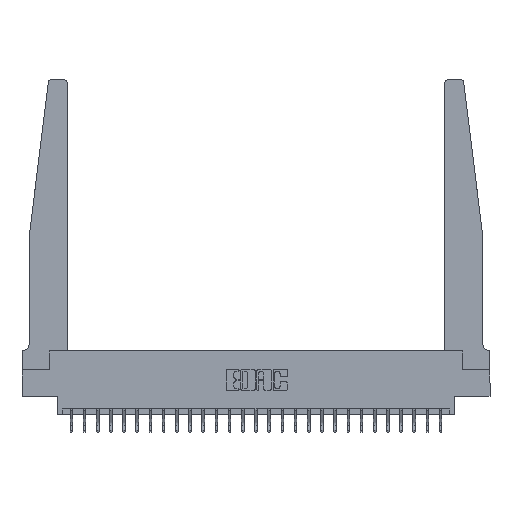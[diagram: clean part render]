
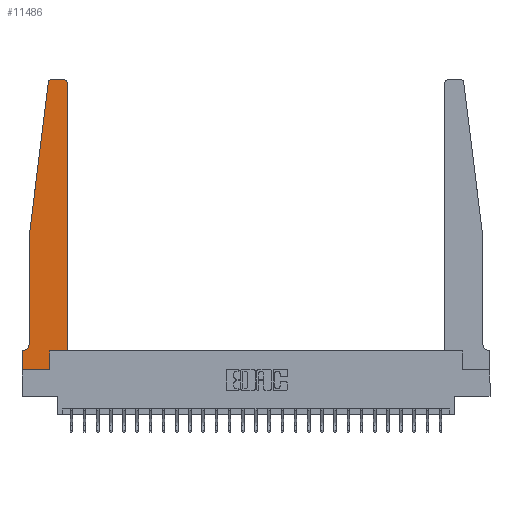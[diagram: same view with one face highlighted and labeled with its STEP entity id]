
A CAD part, top view. The second image highlights one B-rep face of the part: STEP entity #11486.
In plain terms, the highlighted planar face has unit normal (0, 0, 1).
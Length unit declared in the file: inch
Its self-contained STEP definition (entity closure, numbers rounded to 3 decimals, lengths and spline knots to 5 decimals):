
#249 = DIRECTION ( 'NONE',  ( -0.122, -0.992, 0. ) ) ;
#264 = CARTESIAN_POINT ( 'NONE',  ( 0.425, 2.72, 0.37 ) ) ;
#362 = CIRCLE ( 'NONE', #21996, 0.03 ) ;
#432 = VERTEX_POINT ( 'NONE', #3271 ) ;
#933 = EDGE_CURVE ( 'NONE', #6069, #21700, #21223, .T. ) ;
#1213 = CARTESIAN_POINT ( 'NONE',  ( 0., 0., 0.37 ) ) ;
#1563 = CARTESIAN_POINT ( 'NONE',  ( 0., 0.1875, 0.37 ) ) ;
#1593 = VECTOR ( 'NONE', #4755, 39.37008 ) ;
#2114 = CARTESIAN_POINT ( 'NONE',  ( 0.015, 0.2375, 0.37 ) ) ;
#2241 = DIRECTION ( 'NONE',  ( -1., 0., 0. ) ) ;
#2363 = CARTESIAN_POINT ( 'NONE',  ( 0.27653, 2.75, 0.37 ) ) ;
#3149 = EDGE_CURVE ( 'NONE', #21700, #11894, #8370, .T. ) ;
#3271 = CARTESIAN_POINT ( 'NONE',  ( 0.015, 0.1875, 0.37 ) ) ;
#3493 = LINE ( 'NONE', #17425, #9202 ) ;
#4405 = CARTESIAN_POINT ( 'NONE',  ( 0., 0., 0.37 ) ) ;
#4529 = CARTESIAN_POINT ( 'NONE',  ( 0.24675, 2.72367, 0.37 ) ) ;
#4569 = CARTESIAN_POINT ( 'NONE',  ( 0.395, 2.75, 0.37 ) ) ;
#4633 = ORIENTED_EDGE ( 'NONE', *, *, #18553, .T. ) ;
#4755 = DIRECTION ( 'NONE',  ( 0., -1., 0. ) ) ;
#5400 = DIRECTION ( 'NONE',  ( 0., 0., 1. ) ) ;
#5846 = DIRECTION ( 'NONE',  ( -1., 0., 0. ) ) ;
#5895 = EDGE_CURVE ( 'NONE', #11894, #22010, #13922, .T. ) ;
#6009 = ORIENTED_EDGE ( 'NONE', *, *, #15070, .T. ) ;
#6069 = VERTEX_POINT ( 'NONE', #2363 ) ;
#6089 = LINE ( 'NONE', #7996, #8494 ) ;
#6152 = LINE ( 'NONE', #4405, #11100 ) ;
#6614 = PLANE ( 'NONE',  #17190 ) ;
#6619 = VECTOR ( 'NONE', #5846, 39.37008 ) ;
#7009 = DIRECTION ( 'NONE',  ( 1., 0., 0. ) ) ;
#7010 = DIRECTION ( 'NONE',  ( 1., 0., 0. ) ) ;
#7278 = ORIENTED_EDGE ( 'NONE', *, *, #3149, .T. ) ;
#7462 = ORIENTED_EDGE ( 'NONE', *, *, #16626, .T. ) ;
#7742 = ORIENTED_EDGE ( 'NONE', *, *, #25185, .T. ) ;
#7839 = CARTESIAN_POINT ( 'NONE',  ( 0.065, 1.25, 0.37 ) ) ;
#7916 = VERTEX_POINT ( 'NONE', #17795 ) ;
#7996 = CARTESIAN_POINT ( 'NONE',  ( 0.425, 0.18, 0.37 ) ) ;
#8106 = CARTESIAN_POINT ( 'NONE',  ( 0.2605, 0.18, 0.37 ) ) ;
#8370 = LINE ( 'NONE', #24284, #15602 ) ;
#8445 = DIRECTION ( 'NONE',  ( 1., 0., 0. ) ) ;
#8494 = VECTOR ( 'NONE', #24021, 39.37008 ) ;
#8877 = CARTESIAN_POINT ( 'NONE',  ( 0., 0.1875, 0.37 ) ) ;
#9202 = VECTOR ( 'NONE', #25544, 39.37008 ) ;
#9609 = ORIENTED_EDGE ( 'NONE', *, *, #9848, .T. ) ;
#9671 = EDGE_CURVE ( 'NONE', #22010, #432, #14355, .T. ) ;
#9848 = EDGE_CURVE ( 'NONE', #12350, #13671, #22965, .T. ) ;
#10518 = ORIENTED_EDGE ( 'NONE', *, *, #16429, .T. ) ;
#11100 = VECTOR ( 'NONE', #14232, 39.37008 ) ;
#11486 = ADVANCED_FACE ( 'NONE', ( #24807 ), #6614, .T. ) ;
#11536 = ORIENTED_EDGE ( 'NONE', *, *, #933, .T. ) ;
#11894 = VERTEX_POINT ( 'NONE', #7839 ) ;
#12350 = VERTEX_POINT ( 'NONE', #1563 ) ;
#12905 = ORIENTED_EDGE ( 'NONE', *, *, #5895, .T. ) ;
#13084 = CARTESIAN_POINT ( 'NONE',  ( 0.425, 0.18, 0.37 ) ) ;
#13093 = AXIS2_PLACEMENT_3D ( 'NONE', #2114, #14461, #2241 ) ;
#13671 = VERTEX_POINT ( 'NONE', #1213 ) ;
#13922 = LINE ( 'NONE', #24031, #18683 ) ;
#14041 = DIRECTION ( 'NONE',  ( 0., 1., 0. ) ) ;
#14232 = DIRECTION ( 'NONE',  ( 1., 0., 0. ) ) ;
#14243 = DIRECTION ( 'NONE',  ( 0., 0., 1. ) ) ;
#14355 = CIRCLE ( 'NONE', #13093, 0.05 ) ;
#14461 = DIRECTION ( 'NONE',  ( 0., 0., -1. ) ) ;
#14563 = DIRECTION ( 'NONE',  ( 0., 0., 1. ) ) ;
#15070 = EDGE_CURVE ( 'NONE', #22351, #6069, #23907, .T. ) ;
#15185 = VERTEX_POINT ( 'NONE', #264 ) ;
#15484 = CARTESIAN_POINT ( 'NONE',  ( 0.065, 0.2375, 0.37 ) ) ;
#15602 = VECTOR ( 'NONE', #249, 39.37008 ) ;
#16013 = DIRECTION ( 'NONE',  ( 0., 1., 0. ) ) ;
#16377 = CARTESIAN_POINT ( 'NONE',  ( 0.395, 2.72, 0.37 ) ) ;
#16429 = EDGE_CURVE ( 'NONE', #432, #12350, #3493, .T. ) ;
#16549 = AXIS2_PLACEMENT_3D ( 'NONE', #25584, #5400, #7009 ) ;
#16626 = EDGE_CURVE ( 'NONE', #13671, #24482, #6152, .T. ) ;
#17190 = AXIS2_PLACEMENT_3D ( 'NONE', #8877, #14563, #7010 ) ;
#17360 = ORIENTED_EDGE ( 'NONE', *, *, #25662, .T. ) ;
#17425 = CARTESIAN_POINT ( 'NONE',  ( 0.065, 0.1875, 0.37 ) ) ;
#17592 = LINE ( 'NONE', #17716, #21618 ) ;
#17716 = CARTESIAN_POINT ( 'NONE',  ( 0.425, 0.18, 0.37 ) ) ;
#17795 = CARTESIAN_POINT ( 'NONE',  ( 0.2605, 0.18, 0.37 ) ) ;
#18553 = EDGE_CURVE ( 'NONE', #24482, #7916, #24288, .T. ) ;
#18683 = VECTOR ( 'NONE', #25897, 39.37008 ) ;
#19016 = EDGE_CURVE ( 'NONE', #15185, #22351, #362, .T. ) ;
#19026 = ORIENTED_EDGE ( 'NONE', *, *, #9671, .T. ) ;
#19089 = CARTESIAN_POINT ( 'NONE',  ( 0., 0., 0.37 ) ) ;
#20014 = ORIENTED_EDGE ( 'NONE', *, *, #19016, .T. ) ;
#20176 = EDGE_LOOP ( 'NONE', ( #6009, #11536, #7278, #12905, #19026, #10518, #9609, #7462, #4633, #7742, #17360, #20014 ) ) ;
#21223 = CIRCLE ( 'NONE', #16549, 0.03 ) ;
#21618 = VECTOR ( 'NONE', #16013, 39.37008 ) ;
#21700 = VERTEX_POINT ( 'NONE', #4529 ) ;
#21996 = AXIS2_PLACEMENT_3D ( 'NONE', #16377, #14243, #8445 ) ;
#22010 = VERTEX_POINT ( 'NONE', #15484 ) ;
#22351 = VERTEX_POINT ( 'NONE', #4569 ) ;
#22965 = LINE ( 'NONE', #19089, #1593 ) ;
#23261 = VECTOR ( 'NONE', #14041, 39.37008 ) ;
#23519 = CARTESIAN_POINT ( 'NONE',  ( 0.25, 2.75, 0.37 ) ) ;
#23594 = VERTEX_POINT ( 'NONE', #13084 ) ;
#23907 = LINE ( 'NONE', #23519, #6619 ) ;
#24021 = DIRECTION ( 'NONE',  ( 1., 0., 0. ) ) ;
#24031 = CARTESIAN_POINT ( 'NONE',  ( 0.065, 1.25, 0.37 ) ) ;
#24284 = CARTESIAN_POINT ( 'NONE',  ( 0.065, 1.25, 0.37 ) ) ;
#24288 = LINE ( 'NONE', #8106, #23261 ) ;
#24482 = VERTEX_POINT ( 'NONE', #24778 ) ;
#24778 = CARTESIAN_POINT ( 'NONE',  ( 0.2605, 0., 0.37 ) ) ;
#24807 = FACE_OUTER_BOUND ( 'NONE', #20176, .T. ) ;
#25185 = EDGE_CURVE ( 'NONE', #7916, #23594, #6089, .T. ) ;
#25544 = DIRECTION ( 'NONE',  ( -1., 0., 0. ) ) ;
#25584 = CARTESIAN_POINT ( 'NONE',  ( 0.27653, 2.72, 0.37 ) ) ;
#25662 = EDGE_CURVE ( 'NONE', #23594, #15185, #17592, .T. ) ;
#25897 = DIRECTION ( 'NONE',  ( 0., -1., 0. ) ) ;
